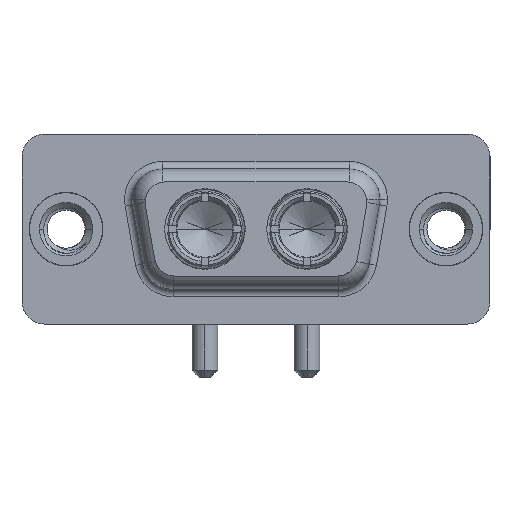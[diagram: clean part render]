
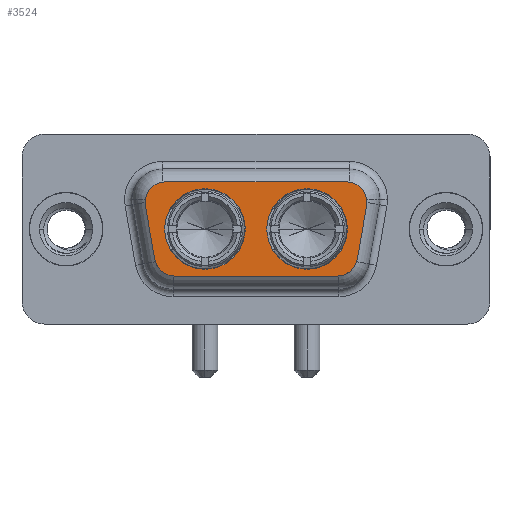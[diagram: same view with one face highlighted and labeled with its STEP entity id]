
A CAD part, top view. The second image highlights one B-rep face of the part: STEP entity #3524.
In plain terms, the highlighted planar face has unit normal (0, 0, 1).
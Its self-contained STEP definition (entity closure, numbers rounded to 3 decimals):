
#82 = EDGE_CURVE ( 'NONE', #3698, #6496, #8960, .T. ) ;
#127 = ORIENTED_EDGE ( 'NONE', *, *, #226, .F. ) ;
#129 = DIRECTION ( 'NONE',  ( -1., 0., 0. ) ) ;
#141 = CARTESIAN_POINT ( 'NONE',  ( 13.21, 0., 6.2 ) ) ;
#226 = EDGE_CURVE ( 'NONE', #9543, #2081, #5636, .T. ) ;
#594 = EDGE_CURVE ( 'NONE', #5390, #4006, #1844, .T. ) ;
#609 = CIRCLE ( 'NONE', #7494, 2.65 ) ;
#648 = CIRCLE ( 'NONE', #3189, 2.65 ) ;
#657 = FACE_OUTER_BOUND ( 'NONE', #7670, .T. ) ;
#660 = DIRECTION ( 'NONE',  ( 0., 0., 1. ) ) ;
#777 = CARTESIAN_POINT ( 'NONE',  ( 7.167, -1.75, 6.2 ) ) ;
#840 = DIRECTION ( 'NONE',  ( -1., 0., 0. ) ) ;
#1220 = CIRCLE ( 'NONE', #10849, 1.35 ) ;
#1295 = ORIENTED_EDGE ( 'NONE', *, *, #3830, .T. ) ;
#1395 = DIRECTION ( 'NONE',  ( 0.174, -0.985, 0. ) ) ;
#1513 = DIRECTION ( 'NONE',  ( 1., 0., 0. ) ) ;
#1547 = CARTESIAN_POINT ( 'NONE',  ( 11.79, 0., 6.2 ) ) ;
#1844 = LINE ( 'NONE', #7455, #6996 ) ;
#2081 = VERTEX_POINT ( 'NONE', #1547 ) ;
#2411 = EDGE_CURVE ( 'NONE', #12084, #5394, #7877, .T. ) ;
#2471 = AXIS2_PLACEMENT_3D ( 'NONE', #5457, #2770, #3513 ) ;
#2497 = FACE_BOUND ( 'NONE', #5484, .T. ) ;
#2550 = EDGE_CURVE ( 'NONE', #11188, #4630, #7728, .T. ) ;
#2770 = DIRECTION ( 'NONE',  ( 0., 0., 1. ) ) ;
#2845 = ORIENTED_EDGE ( 'NONE', *, *, #3295, .T. ) ;
#2927 = CARTESIAN_POINT ( 'NONE',  ( 5.221, 1.516, 6.2 ) ) ;
#3189 = AXIS2_PLACEMENT_3D ( 'NONE', #7786, #11506, #11562 ) ;
#3295 = EDGE_CURVE ( 'NONE', #7605, #3698, #7982, .T. ) ;
#3368 = CIRCLE ( 'NONE', #11613, 1.35 ) ;
#3469 = ORIENTED_EDGE ( 'NONE', *, *, #594, .T. ) ;
#3513 = DIRECTION ( 'NONE',  ( 1., 0., 0. ) ) ;
#3524 = ADVANCED_FACE ( 'NONE', ( #11901, #2497, #657 ), #4478, .F. ) ;
#3558 = DIRECTION ( 'NONE',  ( 1., 0., 0. ) ) ;
#3698 = VERTEX_POINT ( 'NONE', #11278 ) ;
#3830 = EDGE_CURVE ( 'NONE', #5870, #8507, #6803, .T. ) ;
#3933 = ORIENTED_EDGE ( 'NONE', *, *, #8882, .T. ) ;
#4006 = VERTEX_POINT ( 'NONE', #4278 ) ;
#4278 = CARTESIAN_POINT ( 'NONE',  ( 17.833, -3.1, 6.2 ) ) ;
#4478 = PLANE ( 'NONE',  #8571 ) ;
#4480 = DIRECTION ( 'NONE',  ( -1., 0., 0. ) ) ;
#4481 = CIRCLE ( 'NONE', #8795, 1.35 ) ;
#4630 = VERTEX_POINT ( 'NONE', #5091 ) ;
#4772 = AXIS2_PLACEMENT_3D ( 'NONE', #9153, #11169, #8354 ) ;
#4811 = DIRECTION ( 'NONE',  ( 0., 0., 1. ) ) ;
#5091 = CARTESIAN_POINT ( 'NONE',  ( 18.51, 0., 6.2 ) ) ;
#5138 = CARTESIAN_POINT ( 'NONE',  ( 6.49, 0., 6.2 ) ) ;
#5227 = CARTESIAN_POINT ( 'NONE',  ( 9.14, 0., 6.2 ) ) ;
#5315 = EDGE_LOOP ( 'NONE', ( #10710, #11751 ) ) ;
#5378 = ORIENTED_EDGE ( 'NONE', *, *, #6119, .T. ) ;
#5388 = VECTOR ( 'NONE', #1395, 1000. ) ;
#5390 = VERTEX_POINT ( 'NONE', #9005 ) ;
#5394 = VERTEX_POINT ( 'NONE', #8884 ) ;
#5410 = DIRECTION ( 'NONE',  ( -1., 0., 0. ) ) ;
#5457 = CARTESIAN_POINT ( 'NONE',  ( 6.55, 1.75, 6.2 ) ) ;
#5484 = EDGE_LOOP ( 'NONE', ( #11863, #127 ) ) ;
#5636 = CIRCLE ( 'NONE', #10133, 2.65 ) ;
#5671 = CARTESIAN_POINT ( 'NONE',  ( 6.55, 1.75, 6.2 ) ) ;
#5740 = CARTESIAN_POINT ( 'NONE',  ( 18.45, 1.75, 6.2 ) ) ;
#5804 = CARTESIAN_POINT ( 'NONE',  ( 18.45, 3.1, 6.2 ) ) ;
#5851 = DIRECTION ( 'NONE',  ( 1., 0., 0. ) ) ;
#5870 = VERTEX_POINT ( 'NONE', #8866 ) ;
#6058 = DIRECTION ( 'NONE',  ( 0., 0., 1. ) ) ;
#6119 = EDGE_CURVE ( 'NONE', #8507, #7605, #8672, .T. ) ;
#6496 = VERTEX_POINT ( 'NONE', #8472 ) ;
#6622 = ORIENTED_EDGE ( 'NONE', *, *, #8641, .T. ) ;
#6803 = LINE ( 'NONE', #7800, #11390 ) ;
#6996 = VECTOR ( 'NONE', #3558, 1000. ) ;
#7016 = DIRECTION ( 'NONE',  ( -1., 0., 0. ) ) ;
#7168 = VECTOR ( 'NONE', #5410, 1000. ) ;
#7182 = CARTESIAN_POINT ( 'NONE',  ( 17.833, -1.75, 6.2 ) ) ;
#7455 = CARTESIAN_POINT ( 'NONE',  ( 17.833, -3.1, 6.2 ) ) ;
#7494 = AXIS2_PLACEMENT_3D ( 'NONE', #5227, #9936, #1513 ) ;
#7595 = DIRECTION ( 'NONE',  ( 0., 0., 1. ) ) ;
#7605 = VERTEX_POINT ( 'NONE', #5804 ) ;
#7670 = EDGE_LOOP ( 'NONE', ( #7890, #3469, #3933, #1295, #5378, #2845, #11676, #6622, #8658 ) ) ;
#7721 = DIRECTION ( 'NONE',  ( 1., 0., 0. ) ) ;
#7728 = CIRCLE ( 'NONE', #4772, 2.65 ) ;
#7786 = CARTESIAN_POINT ( 'NONE',  ( 15.86, 0., 6.2 ) ) ;
#7800 = CARTESIAN_POINT ( 'NONE',  ( 19.779, 1.516, 6.2 ) ) ;
#7851 = EDGE_CURVE ( 'NONE', #2081, #9543, #609, .T. ) ;
#7877 = LINE ( 'NONE', #8911, #5388 ) ;
#7890 = ORIENTED_EDGE ( 'NONE', *, *, #11342, .T. ) ;
#7982 = LINE ( 'NONE', #9079, #7168 ) ;
#8233 = DIRECTION ( 'NONE',  ( 0., 0., -1. ) ) ;
#8354 = DIRECTION ( 'NONE',  ( 1., 0., 0. ) ) ;
#8472 = CARTESIAN_POINT ( 'NONE',  ( 5.2, 1.75, 6.2 ) ) ;
#8507 = VERTEX_POINT ( 'NONE', #9158 ) ;
#8571 = AXIS2_PLACEMENT_3D ( 'NONE', #777, #8233, #840 ) ;
#8641 = EDGE_CURVE ( 'NONE', #6496, #12084, #3368, .T. ) ;
#8658 = ORIENTED_EDGE ( 'NONE', *, *, #2411, .T. ) ;
#8672 = CIRCLE ( 'NONE', #12002, 1.35 ) ;
#8795 = AXIS2_PLACEMENT_3D ( 'NONE', #11438, #6058, #7016 ) ;
#8866 = CARTESIAN_POINT ( 'NONE',  ( 19.162, -1.984, 6.2 ) ) ;
#8882 = EDGE_CURVE ( 'NONE', #4006, #5870, #1220, .T. ) ;
#8884 = CARTESIAN_POINT ( 'NONE',  ( 5.838, -1.984, 6.2 ) ) ;
#8911 = CARTESIAN_POINT ( 'NONE',  ( 5.838, -1.984, 6.2 ) ) ;
#8960 = CIRCLE ( 'NONE', #2471, 1.35 ) ;
#9005 = CARTESIAN_POINT ( 'NONE',  ( 7.167, -3.1, 6.2 ) ) ;
#9079 = CARTESIAN_POINT ( 'NONE',  ( 6.55, 3.1, 6.2 ) ) ;
#9153 = CARTESIAN_POINT ( 'NONE',  ( 15.86, 0., 6.2 ) ) ;
#9158 = CARTESIAN_POINT ( 'NONE',  ( 19.779, 1.516, 6.2 ) ) ;
#9399 = DIRECTION ( 'NONE',  ( 0., 0., 1. ) ) ;
#9493 = CARTESIAN_POINT ( 'NONE',  ( 9.14, 0., 6.2 ) ) ;
#9543 = VERTEX_POINT ( 'NONE', #5138 ) ;
#9626 = EDGE_CURVE ( 'NONE', #4630, #11188, #648, .T. ) ;
#9936 = DIRECTION ( 'NONE',  ( 0., 0., 1. ) ) ;
#10133 = AXIS2_PLACEMENT_3D ( 'NONE', #9493, #7595, #7721 ) ;
#10667 = DIRECTION ( 'NONE',  ( 0.174, 0.985, 0. ) ) ;
#10710 = ORIENTED_EDGE ( 'NONE', *, *, #9626, .F. ) ;
#10849 = AXIS2_PLACEMENT_3D ( 'NONE', #7182, #660, #4480 ) ;
#11169 = DIRECTION ( 'NONE',  ( 0., 0., 1. ) ) ;
#11188 = VERTEX_POINT ( 'NONE', #141 ) ;
#11278 = CARTESIAN_POINT ( 'NONE',  ( 6.55, 3.1, 6.2 ) ) ;
#11342 = EDGE_CURVE ( 'NONE', #5394, #5390, #4481, .T. ) ;
#11390 = VECTOR ( 'NONE', #10667, 1000. ) ;
#11438 = CARTESIAN_POINT ( 'NONE',  ( 7.167, -1.75, 6.2 ) ) ;
#11506 = DIRECTION ( 'NONE',  ( 0., 0., 1. ) ) ;
#11562 = DIRECTION ( 'NONE',  ( 1., 0., 0. ) ) ;
#11613 = AXIS2_PLACEMENT_3D ( 'NONE', #5671, #9399, #5851 ) ;
#11676 = ORIENTED_EDGE ( 'NONE', *, *, #82, .T. ) ;
#11751 = ORIENTED_EDGE ( 'NONE', *, *, #2550, .F. ) ;
#11863 = ORIENTED_EDGE ( 'NONE', *, *, #7851, .F. ) ;
#11901 = FACE_BOUND ( 'NONE', #5315, .T. ) ;
#12002 = AXIS2_PLACEMENT_3D ( 'NONE', #5740, #4811, #129 ) ;
#12084 = VERTEX_POINT ( 'NONE', #2927 ) ;
